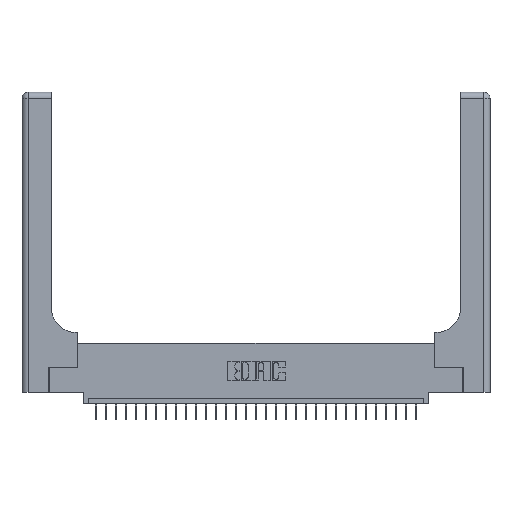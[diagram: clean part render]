
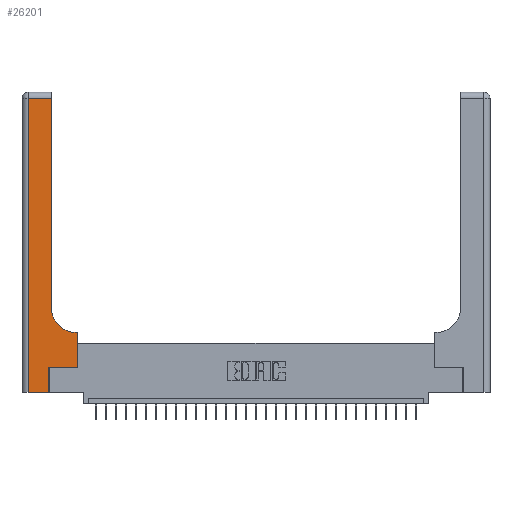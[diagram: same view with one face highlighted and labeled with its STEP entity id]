
A CAD part, top view. The second image highlights one B-rep face of the part: STEP entity #26201.
In plain terms, the highlighted planar face has unit normal (0, 0, 1).
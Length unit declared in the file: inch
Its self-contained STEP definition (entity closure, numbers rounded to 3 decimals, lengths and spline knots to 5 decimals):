
#424 = CARTESIAN_POINT ( 'NONE',  ( 0., 0., 0.37 ) ) ;
#1034 = VERTEX_POINT ( 'NONE', #9822 ) ;
#1738 = CIRCLE ( 'NONE', #21804, 0.25 ) ;
#2043 = VECTOR ( 'NONE', #12646, 39.37008 ) ;
#3672 = ORIENTED_EDGE ( 'NONE', *, *, #30947, .T. ) ;
#3697 = ORIENTED_EDGE ( 'NONE', *, *, #4544, .T. ) ;
#3838 = CARTESIAN_POINT ( 'NONE',  ( 0.06, 3., 0.37 ) ) ;
#3902 = LINE ( 'NONE', #3838, #5779 ) ;
#4148 = DIRECTION ( 'NONE',  ( 0., 1., 0. ) ) ;
#4544 = EDGE_CURVE ( 'NONE', #26323, #26207, #10966, .T. ) ;
#5779 = VECTOR ( 'NONE', #28080, 39.37008 ) ;
#6848 = CARTESIAN_POINT ( 'NONE',  ( 0.5585, 0.25, 0.37 ) ) ;
#7098 = VERTEX_POINT ( 'NONE', #10447 ) ;
#7404 = ORIENTED_EDGE ( 'NONE', *, *, #8417, .T. ) ;
#7954 = EDGE_CURVE ( 'NONE', #28216, #7098, #19867, .T. ) ;
#8211 = CARTESIAN_POINT ( 'NONE',  ( 0.269, 0., 0.37 ) ) ;
#8339 = DIRECTION ( 'NONE',  ( 1., 0., 0. ) ) ;
#8417 = EDGE_CURVE ( 'NONE', #9314, #1034, #24328, .T. ) ;
#8553 = DIRECTION ( 'NONE',  ( -1., 0., 0. ) ) ;
#8715 = ORIENTED_EDGE ( 'NONE', *, *, #29306, .T. ) ;
#9314 = VERTEX_POINT ( 'NONE', #12926 ) ;
#9439 = EDGE_CURVE ( 'NONE', #14491, #26323, #21257, .T. ) ;
#9570 = CARTESIAN_POINT ( 'NONE',  ( 0.269, 0.25, 0.37 ) ) ;
#9822 = CARTESIAN_POINT ( 'NONE',  ( 0.2915, 2.94, 0.37 ) ) ;
#9939 = EDGE_CURVE ( 'NONE', #7098, #14491, #25366, .T. ) ;
#10447 = CARTESIAN_POINT ( 'NONE',  ( 0.269, 0., 0.37 ) ) ;
#10896 = EDGE_CURVE ( 'NONE', #1034, #15608, #13361, .T. ) ;
#10966 = LINE ( 'NONE', #6848, #23041 ) ;
#12646 = DIRECTION ( 'NONE',  ( 1., 0., 0. ) ) ;
#12926 = CARTESIAN_POINT ( 'NONE',  ( 0.2915, 0.85, 0.37 ) ) ;
#13361 = LINE ( 'NONE', #22809, #22818 ) ;
#14491 = VERTEX_POINT ( 'NONE', #28211 ) ;
#14750 = DIRECTION ( 'NONE',  ( 0., 0., -1. ) ) ;
#15608 = VERTEX_POINT ( 'NONE', #21490 ) ;
#16577 = CARTESIAN_POINT ( 'NONE',  ( 0., 3., 0.37 ) ) ;
#17213 = LINE ( 'NONE', #28348, #27079 ) ;
#17285 = DIRECTION ( 'NONE',  ( -1., 0., 0. ) ) ;
#18659 = CARTESIAN_POINT ( 'NONE',  ( 0.2915, 3., 0.37 ) ) ;
#19357 = CARTESIAN_POINT ( 'NONE',  ( 0.5585, 0.6, 0.37 ) ) ;
#19867 = LINE ( 'NONE', #424, #2043 ) ;
#20263 = ORIENTED_EDGE ( 'NONE', *, *, #9439, .T. ) ;
#20934 = VERTEX_POINT ( 'NONE', #25901 ) ;
#21257 = LINE ( 'NONE', #9570, #28843 ) ;
#21490 = CARTESIAN_POINT ( 'NONE',  ( 0.06, 2.94, 0.37 ) ) ;
#21701 = DIRECTION ( 'NONE',  ( 0., 1., 0. ) ) ;
#21804 = AXIS2_PLACEMENT_3D ( 'NONE', #29963, #30074, #8339 ) ;
#22497 = DIRECTION ( 'NONE',  ( 1., 0., 0. ) ) ;
#22809 = CARTESIAN_POINT ( 'NONE',  ( 0., 2.94, 0.37 ) ) ;
#22818 = VECTOR ( 'NONE', #8553, 39.37008 ) ;
#23041 = VECTOR ( 'NONE', #21701, 39.37008 ) ;
#23535 = ORIENTED_EDGE ( 'NONE', *, *, #7954, .T. ) ;
#23760 = PLANE ( 'NONE',  #29673 ) ;
#23970 = CARTESIAN_POINT ( 'NONE',  ( 0.5585, 0.25, 0.37 ) ) ;
#24260 = EDGE_CURVE ( 'NONE', #15608, #28216, #3902, .T. ) ;
#24328 = LINE ( 'NONE', #18659, #29296 ) ;
#24576 = FACE_OUTER_BOUND ( 'NONE', #26988, .T. ) ;
#24608 = VECTOR ( 'NONE', #25014, 39.37008 ) ;
#25014 = DIRECTION ( 'NONE',  ( 0., 1., 0. ) ) ;
#25366 = LINE ( 'NONE', #8211, #24608 ) ;
#25881 = DIRECTION ( 'NONE',  ( -1., 0., 0. ) ) ;
#25901 = CARTESIAN_POINT ( 'NONE',  ( 0.5415, 0.6, 0.37 ) ) ;
#26201 = ADVANCED_FACE ( 'NONE', ( #24576 ), #23760, .F. ) ;
#26207 = VERTEX_POINT ( 'NONE', #19357 ) ;
#26323 = VERTEX_POINT ( 'NONE', #23970 ) ;
#26481 = ORIENTED_EDGE ( 'NONE', *, *, #10896, .T. ) ;
#26988 = EDGE_LOOP ( 'NONE', ( #7404, #26481, #27482, #23535, #31303, #20263, #3697, #8715, #3672 ) ) ;
#27079 = VECTOR ( 'NONE', #25881, 39.37008 ) ;
#27482 = ORIENTED_EDGE ( 'NONE', *, *, #24260, .T. ) ;
#28080 = DIRECTION ( 'NONE',  ( 0., -1., 0. ) ) ;
#28211 = CARTESIAN_POINT ( 'NONE',  ( 0.269, 0.25, 0.37 ) ) ;
#28216 = VERTEX_POINT ( 'NONE', #30549 ) ;
#28348 = CARTESIAN_POINT ( 'NONE',  ( 0.2915, 0.6, 0.37 ) ) ;
#28843 = VECTOR ( 'NONE', #22497, 39.37008 ) ;
#29296 = VECTOR ( 'NONE', #4148, 39.37008 ) ;
#29306 = EDGE_CURVE ( 'NONE', #26207, #20934, #17213, .T. ) ;
#29673 = AXIS2_PLACEMENT_3D ( 'NONE', #16577, #14750, #17285 ) ;
#29963 = CARTESIAN_POINT ( 'NONE',  ( 0.5415, 0.85, 0.37 ) ) ;
#30074 = DIRECTION ( 'NONE',  ( 0., 0., -1. ) ) ;
#30549 = CARTESIAN_POINT ( 'NONE',  ( 0.06, 0., 0.37 ) ) ;
#30947 = EDGE_CURVE ( 'NONE', #20934, #9314, #1738, .T. ) ;
#31303 = ORIENTED_EDGE ( 'NONE', *, *, #9939, .T. ) ;
